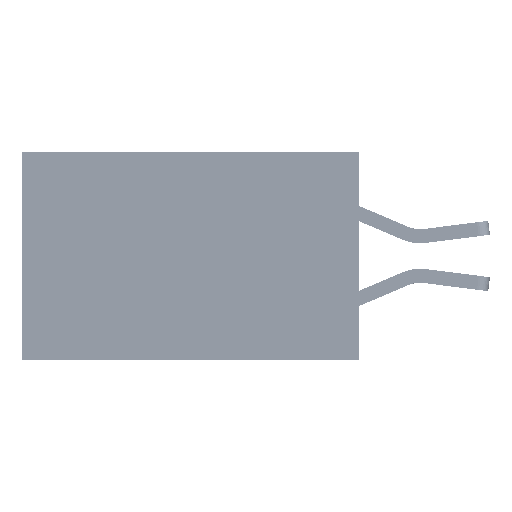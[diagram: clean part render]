
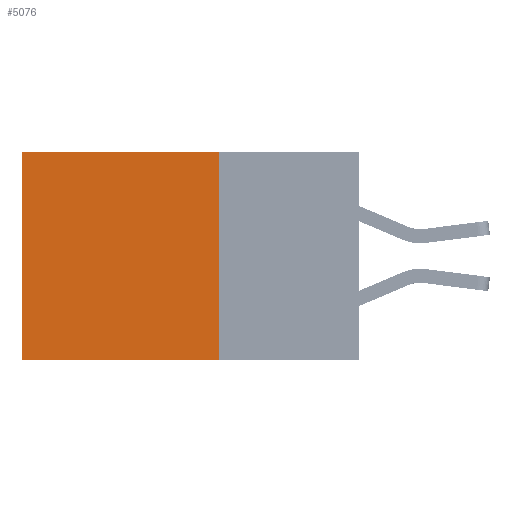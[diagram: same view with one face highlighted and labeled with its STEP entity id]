
A CAD part, left-side view. The second image highlights one B-rep face of the part: STEP entity #5076.
In plain terms, the highlighted planar face has unit normal (-1, 0, 0).
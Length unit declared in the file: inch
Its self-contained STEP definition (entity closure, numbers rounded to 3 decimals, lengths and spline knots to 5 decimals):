
#740 = VECTOR ( 'NONE', #9214, 39.37008 ) ;
#767 = VERTEX_POINT ( 'NONE', #38948 ) ;
#843 = ORIENTED_EDGE ( 'NONE', *, *, #3019, .F. ) ;
#1324 = CARTESIAN_POINT ( 'NONE',  ( 0.2875, 0.25, 0. ) ) ;
#3019 = EDGE_CURVE ( 'NONE', #20901, #19116, #17949, .T. ) ;
#4914 = VECTOR ( 'NONE', #33095, 39.37008 ) ;
#5076 = ADVANCED_FACE ( 'NONE', ( #15892 ), #11999, .F. ) ;
#5655 = CARTESIAN_POINT ( 'NONE',  ( 0.2875, 0.25, 0. ) ) ;
#8103 = LINE ( 'NONE', #5655, #27373 ) ;
#9214 = DIRECTION ( 'NONE',  ( 0., 0., -1. ) ) ;
#9333 = DIRECTION ( 'NONE',  ( 0., 1., 0. ) ) ;
#11351 = LINE ( 'NONE', #24039, #740 ) ;
#11512 = ORIENTED_EDGE ( 'NONE', *, *, #17101, .T. ) ;
#11602 = CARTESIAN_POINT ( 'NONE',  ( 0.2875, 0.6, -0.37 ) ) ;
#11999 = PLANE ( 'NONE',  #24199 ) ;
#15583 = ORIENTED_EDGE ( 'NONE', *, *, #34454, .T. ) ;
#15629 = EDGE_CURVE ( 'NONE', #20686, #20901, #8103, .T. ) ;
#15659 = LINE ( 'NONE', #24162, #34407 ) ;
#15892 = FACE_OUTER_BOUND ( 'NONE', #16086, .T. ) ;
#16086 = EDGE_LOOP ( 'NONE', ( #15583, #843, #28334, #11512 ) ) ;
#17101 = EDGE_CURVE ( 'NONE', #20686, #767, #15659, .T. ) ;
#17949 = LINE ( 'NONE', #30042, #4914 ) ;
#19116 = VERTEX_POINT ( 'NONE', #11602 ) ;
#20686 = VERTEX_POINT ( 'NONE', #1324 ) ;
#20901 = VERTEX_POINT ( 'NONE', #36400 ) ;
#24039 = CARTESIAN_POINT ( 'NONE',  ( 0.2875, 0.6, 0. ) ) ;
#24162 = CARTESIAN_POINT ( 'NONE',  ( 0.2875, 0.25, 0. ) ) ;
#24199 = AXIS2_PLACEMENT_3D ( 'NONE', #24547, #24411, #36972 ) ;
#24411 = DIRECTION ( 'NONE',  ( 1., 0., 0. ) ) ;
#24547 = CARTESIAN_POINT ( 'NONE',  ( 0.2875, 0.25, 0. ) ) ;
#26955 = DIRECTION ( 'NONE',  ( 0., 0., -1. ) ) ;
#27373 = VECTOR ( 'NONE', #26955, 39.37008 ) ;
#28334 = ORIENTED_EDGE ( 'NONE', *, *, #15629, .F. ) ;
#30042 = CARTESIAN_POINT ( 'NONE',  ( 0.2875, 0.25, -0.37 ) ) ;
#33095 = DIRECTION ( 'NONE',  ( 0., 1., 0. ) ) ;
#34407 = VECTOR ( 'NONE', #9333, 39.37008 ) ;
#34454 = EDGE_CURVE ( 'NONE', #767, #19116, #11351, .T. ) ;
#36400 = CARTESIAN_POINT ( 'NONE',  ( 0.2875, 0.25, -0.37 ) ) ;
#36972 = DIRECTION ( 'NONE',  ( 0., 0., -1. ) ) ;
#38948 = CARTESIAN_POINT ( 'NONE',  ( 0.2875, 0.6, 0. ) ) ;
